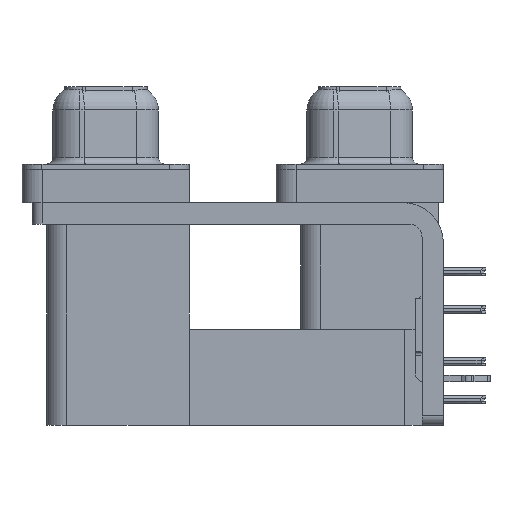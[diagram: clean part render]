
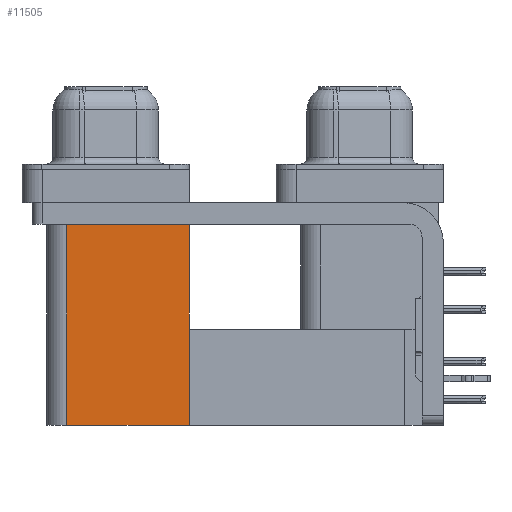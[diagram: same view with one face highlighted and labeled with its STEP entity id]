
A CAD part, left-side view. The second image highlights one B-rep face of the part: STEP entity #11505.
In plain terms, the highlighted planar face has unit normal (-1, 0, 0).
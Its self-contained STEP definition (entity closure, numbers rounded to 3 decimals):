
#4627 = FACE_OUTER_BOUND ( 'NONE', #9005, .T. ) ;
#6941 = EDGE_CURVE ( 'NONE', #8604, #45778, #46551, .T. ) ;
#7115 = CARTESIAN_POINT ( 'NONE',  ( 3.765, 21.975, -19.2 ) ) ;
#8604 = VERTEX_POINT ( 'NONE', #20629 ) ;
#9005 = EDGE_LOOP ( 'NONE', ( #27317, #35745, #27145, #27817 ) ) ;
#11505 = ADVANCED_FACE ( 'NONE', ( #4627 ), #45904, .F. ) ;
#12449 = DIRECTION ( 'NONE',  ( 1., 0., 0. ) ) ;
#18745 = VECTOR ( 'NONE', #34617, 1000. ) ;
#18776 = VECTOR ( 'NONE', #44479, 1000. ) ;
#19058 = LINE ( 'NONE', #34205, #21263 ) ;
#20550 = CARTESIAN_POINT ( 'NONE',  ( 3.765, 21.975, -19.2 ) ) ;
#20629 = CARTESIAN_POINT ( 'NONE',  ( 3.765, 12.775, -19.2 ) ) ;
#21263 = VECTOR ( 'NONE', #26887, 1000. ) ;
#21370 = EDGE_CURVE ( 'NONE', #27395, #30766, #19058, .T. ) ;
#23621 = CARTESIAN_POINT ( 'NONE',  ( 3.765, 12.775, -19.2 ) ) ;
#26128 = CARTESIAN_POINT ( 'NONE',  ( 3.765, 21.975, -2.5 ) ) ;
#26887 = DIRECTION ( 'NONE',  ( 0., 1., 0. ) ) ;
#27145 = ORIENTED_EDGE ( 'NONE', *, *, #6941, .F. ) ;
#27317 = ORIENTED_EDGE ( 'NONE', *, *, #21370, .T. ) ;
#27361 = DIRECTION ( 'NONE',  ( 0., 0., -1. ) ) ;
#27395 = VERTEX_POINT ( 'NONE', #28178 ) ;
#27817 = ORIENTED_EDGE ( 'NONE', *, *, #45187, .T. ) ;
#28178 = CARTESIAN_POINT ( 'NONE',  ( 3.765, 12.775, -2.5 ) ) ;
#30766 = VERTEX_POINT ( 'NONE', #26128 ) ;
#33290 = LINE ( 'NONE', #7115, #18776 ) ;
#34205 = CARTESIAN_POINT ( 'NONE',  ( 3.765, 12.775, -2.5 ) ) ;
#34456 = CARTESIAN_POINT ( 'NONE',  ( 3.765, 12.775, -19.2 ) ) ;
#34617 = DIRECTION ( 'NONE',  ( 0., 0., 1. ) ) ;
#34854 = LINE ( 'NONE', #23621, #18745 ) ;
#35338 = DIRECTION ( 'NONE',  ( 0., 1., 0. ) ) ;
#35745 = ORIENTED_EDGE ( 'NONE', *, *, #45596, .F. ) ;
#38419 = AXIS2_PLACEMENT_3D ( 'NONE', #34456, #12449, #27361 ) ;
#44479 = DIRECTION ( 'NONE',  ( 0., 0., 1. ) ) ;
#45187 = EDGE_CURVE ( 'NONE', #8604, #27395, #34854, .T. ) ;
#45596 = EDGE_CURVE ( 'NONE', #45778, #30766, #33290, .T. ) ;
#45778 = VERTEX_POINT ( 'NONE', #20550 ) ;
#45904 = PLANE ( 'NONE',  #38419 ) ;
#46551 = LINE ( 'NONE', #46773, #47790 ) ;
#46773 = CARTESIAN_POINT ( 'NONE',  ( 3.765, 12.775, -19.2 ) ) ;
#47790 = VECTOR ( 'NONE', #35338, 1000. ) ;
